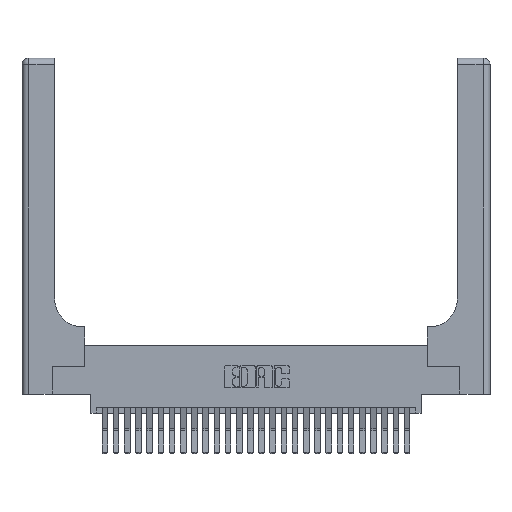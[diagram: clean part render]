
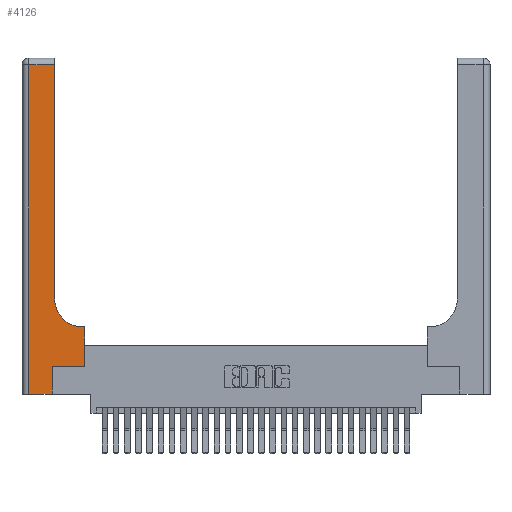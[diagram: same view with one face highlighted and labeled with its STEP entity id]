
A CAD part, top view. The second image highlights one B-rep face of the part: STEP entity #4126.
In plain terms, the highlighted planar face has unit normal (0, 0, 1).
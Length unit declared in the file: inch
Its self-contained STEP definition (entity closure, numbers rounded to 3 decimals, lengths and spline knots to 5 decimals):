
#23 = ORIENTED_EDGE ( 'NONE', *, *, #19432, .T. ) ;
#580 = CARTESIAN_POINT ( 'NONE',  ( 0., 0., 0.37 ) ) ;
#1456 = LINE ( 'NONE', #3038, #6757 ) ;
#1583 = DIRECTION ( 'NONE',  ( 0., 1., 0. ) ) ;
#2433 = VECTOR ( 'NONE', #15284, 39.37008 ) ;
#2589 = ORIENTED_EDGE ( 'NONE', *, *, #6060, .T. ) ;
#2953 = CARTESIAN_POINT ( 'NONE',  ( 0.269, 0.25, 0.37 ) ) ;
#2969 = EDGE_CURVE ( 'NONE', #24940, #28158, #1456, .T. ) ;
#3038 = CARTESIAN_POINT ( 'NONE',  ( 0., 2.94, 0.37 ) ) ;
#3810 = LINE ( 'NONE', #9110, #14406 ) ;
#3922 = LINE ( 'NONE', #4362, #20587 ) ;
#4126 = ADVANCED_FACE ( 'NONE', ( #14158 ), #26168, .F. ) ;
#4362 = CARTESIAN_POINT ( 'NONE',  ( 0.5585, 0.25, 0.37 ) ) ;
#4905 = CARTESIAN_POINT ( 'NONE',  ( 0.5415, 0.85, 0.37 ) ) ;
#6060 = EDGE_CURVE ( 'NONE', #14372, #24940, #15144, .T. ) ;
#6175 = CARTESIAN_POINT ( 'NONE',  ( 0.2915, 3., 0.37 ) ) ;
#6311 = DIRECTION ( 'NONE',  ( 0., -1., 0. ) ) ;
#6459 = LINE ( 'NONE', #24366, #11026 ) ;
#6757 = VECTOR ( 'NONE', #14277, 39.37008 ) ;
#6876 = AXIS2_PLACEMENT_3D ( 'NONE', #4905, #20765, #7163 ) ;
#7163 = DIRECTION ( 'NONE',  ( 1., 0., 0. ) ) ;
#7986 = EDGE_CURVE ( 'NONE', #21446, #17483, #25659, .T. ) ;
#8393 = VERTEX_POINT ( 'NONE', #11889 ) ;
#9110 = CARTESIAN_POINT ( 'NONE',  ( 0.269, 0.25, 0.37 ) ) ;
#9798 = ORIENTED_EDGE ( 'NONE', *, *, #2969, .T. ) ;
#10190 = EDGE_CURVE ( 'NONE', #10579, #14372, #13112, .T. ) ;
#10579 = VERTEX_POINT ( 'NONE', #20243 ) ;
#10736 = CARTESIAN_POINT ( 'NONE',  ( 0.06, 0., 0.37 ) ) ;
#11026 = VECTOR ( 'NONE', #26628, 39.37008 ) ;
#11481 = ORIENTED_EDGE ( 'NONE', *, *, #17440, .T. ) ;
#11889 = CARTESIAN_POINT ( 'NONE',  ( 0.5585, 0.6, 0.37 ) ) ;
#12180 = AXIS2_PLACEMENT_3D ( 'NONE', #23888, #28424, #14877 ) ;
#12253 = LINE ( 'NONE', #580, #12984 ) ;
#12259 = CARTESIAN_POINT ( 'NONE',  ( 0.06, 2.94, 0.37 ) ) ;
#12723 = ORIENTED_EDGE ( 'NONE', *, *, #22310, .T. ) ;
#12984 = VECTOR ( 'NONE', #18685, 39.37008 ) ;
#13112 = CIRCLE ( 'NONE', #6876, 0.25 ) ;
#13424 = VERTEX_POINT ( 'NONE', #23937 ) ;
#13609 = EDGE_CURVE ( 'NONE', #28158, #27021, #14632, .T. ) ;
#14158 = FACE_OUTER_BOUND ( 'NONE', #27354, .T. ) ;
#14277 = DIRECTION ( 'NONE',  ( -1., 0., 0. ) ) ;
#14372 = VERTEX_POINT ( 'NONE', #24789 ) ;
#14406 = VECTOR ( 'NONE', #20460, 39.37008 ) ;
#14632 = LINE ( 'NONE', #17712, #19987 ) ;
#14877 = DIRECTION ( 'NONE',  ( -1., 0., 0. ) ) ;
#15055 = CARTESIAN_POINT ( 'NONE',  ( 0.2915, 2.94, 0.37 ) ) ;
#15144 = LINE ( 'NONE', #6175, #2433 ) ;
#15284 = DIRECTION ( 'NONE',  ( 0., 1., 0. ) ) ;
#15470 = EDGE_CURVE ( 'NONE', #13424, #8393, #3922, .T. ) ;
#17396 = CARTESIAN_POINT ( 'NONE',  ( 0.269, 0., 0.37 ) ) ;
#17440 = EDGE_CURVE ( 'NONE', #27021, #21446, #12253, .T. ) ;
#17483 = VERTEX_POINT ( 'NONE', #2953 ) ;
#17712 = CARTESIAN_POINT ( 'NONE',  ( 0.06, 3., 0.37 ) ) ;
#17923 = DIRECTION ( 'NONE',  ( 0., 1., 0. ) ) ;
#18607 = ORIENTED_EDGE ( 'NONE', *, *, #10190, .T. ) ;
#18685 = DIRECTION ( 'NONE',  ( 1., 0., 0. ) ) ;
#19432 = EDGE_CURVE ( 'NONE', #8393, #10579, #6459, .T. ) ;
#19680 = VECTOR ( 'NONE', #1583, 39.37008 ) ;
#19987 = VECTOR ( 'NONE', #6311, 39.37008 ) ;
#20167 = ORIENTED_EDGE ( 'NONE', *, *, #13609, .T. ) ;
#20243 = CARTESIAN_POINT ( 'NONE',  ( 0.5415, 0.6, 0.37 ) ) ;
#20460 = DIRECTION ( 'NONE',  ( 1., 0., 0. ) ) ;
#20587 = VECTOR ( 'NONE', #17923, 39.37008 ) ;
#20765 = DIRECTION ( 'NONE',  ( 0., 0., -1. ) ) ;
#21313 = ORIENTED_EDGE ( 'NONE', *, *, #7986, .T. ) ;
#21446 = VERTEX_POINT ( 'NONE', #28649 ) ;
#22310 = EDGE_CURVE ( 'NONE', #17483, #13424, #3810, .T. ) ;
#23888 = CARTESIAN_POINT ( 'NONE',  ( 0., 3., 0.37 ) ) ;
#23937 = CARTESIAN_POINT ( 'NONE',  ( 0.5585, 0.25, 0.37 ) ) ;
#24366 = CARTESIAN_POINT ( 'NONE',  ( 0.2915, 0.6, 0.37 ) ) ;
#24748 = ORIENTED_EDGE ( 'NONE', *, *, #15470, .T. ) ;
#24789 = CARTESIAN_POINT ( 'NONE',  ( 0.2915, 0.85, 0.37 ) ) ;
#24940 = VERTEX_POINT ( 'NONE', #15055 ) ;
#25659 = LINE ( 'NONE', #17396, #19680 ) ;
#26168 = PLANE ( 'NONE',  #12180 ) ;
#26628 = DIRECTION ( 'NONE',  ( -1., 0., 0. ) ) ;
#27021 = VERTEX_POINT ( 'NONE', #10736 ) ;
#27354 = EDGE_LOOP ( 'NONE', ( #2589, #9798, #20167, #11481, #21313, #12723, #24748, #23, #18607 ) ) ;
#28158 = VERTEX_POINT ( 'NONE', #12259 ) ;
#28424 = DIRECTION ( 'NONE',  ( 0., 0., -1. ) ) ;
#28649 = CARTESIAN_POINT ( 'NONE',  ( 0.269, 0., 0.37 ) ) ;
